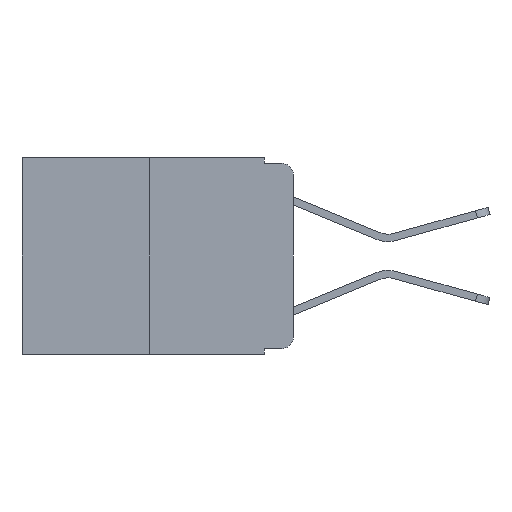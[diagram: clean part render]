
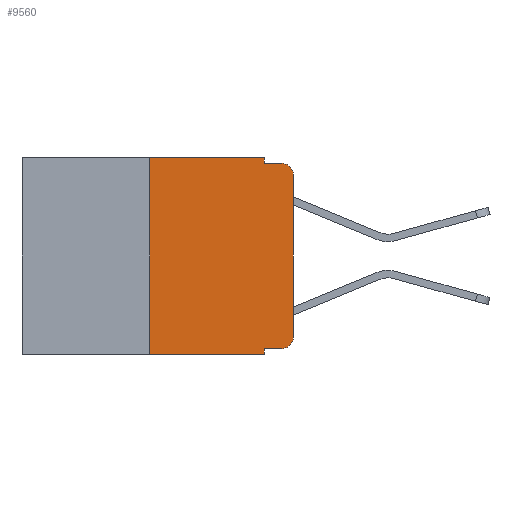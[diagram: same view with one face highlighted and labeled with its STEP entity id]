
A CAD part, left-side view. The second image highlights one B-rep face of the part: STEP entity #9560.
In plain terms, the highlighted planar face has unit normal (-1, 0, 0).
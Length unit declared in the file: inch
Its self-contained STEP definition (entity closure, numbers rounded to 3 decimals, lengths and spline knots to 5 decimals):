
#99 = VECTOR ( 'NONE', #3078, 39.37008 ) ;
#804 = DIRECTION ( 'NONE',  ( 0., -1., 0. ) ) ;
#1243 = ORIENTED_EDGE ( 'NONE', *, *, #24060, .F. ) ;
#1308 = CARTESIAN_POINT ( 'NONE',  ( 0., 0.473, 0. ) ) ;
#1434 = CARTESIAN_POINT ( 'NONE',  ( 0., 0.051, 0. ) ) ;
#1743 = DIRECTION ( 'NONE',  ( 0., 0., -1. ) ) ;
#1775 = DIRECTION ( 'NONE',  ( 0., 0., -1. ) ) ;
#1901 = ORIENTED_EDGE ( 'NONE', *, *, #14329, .F. ) ;
#2066 = VERTEX_POINT ( 'NONE', #2120 ) ;
#2120 = CARTESIAN_POINT ( 'NONE',  ( 0., 0.25, 0. ) ) ;
#2760 = PLANE ( 'NONE',  #17111 ) ;
#3078 = DIRECTION ( 'NONE',  ( 0., 0., 1. ) ) ;
#3568 = DIRECTION ( 'NONE',  ( -1., 0., 0. ) ) ;
#3966 = EDGE_CURVE ( 'NONE', #24525, #5085, #13087, .T. ) ;
#4762 = AXIS2_PLACEMENT_3D ( 'NONE', #24949, #13634, #1775 ) ;
#5085 = VERTEX_POINT ( 'NONE', #5779 ) ;
#5116 = LINE ( 'NONE', #18651, #10377 ) ;
#5595 = VERTEX_POINT ( 'NONE', #20746 ) ;
#5746 = VERTEX_POINT ( 'NONE', #14471 ) ;
#5779 = CARTESIAN_POINT ( 'NONE',  ( 0., 0.051, -0.343 ) ) ;
#5950 = VERTEX_POINT ( 'NONE', #19488 ) ;
#6272 = FACE_OUTER_BOUND ( 'NONE', #22135, .T. ) ;
#6300 = LINE ( 'NONE', #11685, #11519 ) ;
#6375 = LINE ( 'NONE', #20889, #21184 ) ;
#6711 = CARTESIAN_POINT ( 'NONE',  ( 0., 0.02, -0.03 ) ) ;
#6870 = DIRECTION ( 'NONE',  ( 0., 0., -1. ) ) ;
#6965 = DIRECTION ( 'NONE',  ( 0., -1., 0. ) ) ;
#7003 = EDGE_CURVE ( 'NONE', #5746, #5595, #13143, .T. ) ;
#7626 = CARTESIAN_POINT ( 'NONE',  ( 0., 0.25, -0.343 ) ) ;
#7671 = VERTEX_POINT ( 'NONE', #25083 ) ;
#7729 = EDGE_CURVE ( 'NONE', #18114, #5085, #6375, .T. ) ;
#7801 = EDGE_CURVE ( 'NONE', #21538, #5746, #5116, .T. ) ;
#7906 = ORIENTED_EDGE ( 'NONE', *, *, #7801, .T. ) ;
#7924 = VECTOR ( 'NONE', #15656, 39.37008 ) ;
#8271 = VERTEX_POINT ( 'NONE', #12628 ) ;
#8515 = ORIENTED_EDGE ( 'NONE', *, *, #7003, .T. ) ;
#8779 = CARTESIAN_POINT ( 'NONE',  ( 0., 0.051, -0.333 ) ) ;
#9560 = ADVANCED_FACE ( 'NONE', ( #6272 ), #2760, .F. ) ;
#9796 = CARTESIAN_POINT ( 'NONE',  ( 0., 0.051, 0. ) ) ;
#10217 = LINE ( 'NONE', #16835, #99 ) ;
#10377 = VECTOR ( 'NONE', #22731, 39.37008 ) ;
#10652 = ORIENTED_EDGE ( 'NONE', *, *, #15314, .T. ) ;
#11247 = ORIENTED_EDGE ( 'NONE', *, *, #7729, .T. ) ;
#11519 = VECTOR ( 'NONE', #21248, 39.37008 ) ;
#11596 = LINE ( 'NONE', #1308, #16732 ) ;
#11674 = EDGE_CURVE ( 'NONE', #18114, #2066, #10217, .T. ) ;
#11685 = CARTESIAN_POINT ( 'NONE',  ( 0., 0.051, -0.333 ) ) ;
#12448 = ORIENTED_EDGE ( 'NONE', *, *, #17003, .F. ) ;
#12628 = CARTESIAN_POINT ( 'NONE',  ( 0., 0.051, 0. ) ) ;
#12994 = CARTESIAN_POINT ( 'NONE',  ( 0., 0., -0.313 ) ) ;
#13010 = DIRECTION ( 'NONE',  ( 0., 0., -1. ) ) ;
#13087 = LINE ( 'NONE', #1434, #7924 ) ;
#13143 = CIRCLE ( 'NONE', #15792, 0.02 ) ;
#13466 = CIRCLE ( 'NONE', #4762, 0.02 ) ;
#13634 = DIRECTION ( 'NONE',  ( -1., 0., 0. ) ) ;
#14129 = VECTOR ( 'NONE', #804, 39.37008 ) ;
#14329 = EDGE_CURVE ( 'NONE', #7671, #5595, #24170, .T. ) ;
#14471 = CARTESIAN_POINT ( 'NONE',  ( 0., 0., -0.03 ) ) ;
#15148 = DIRECTION ( 'NONE',  ( 0., -1., 0. ) ) ;
#15176 = ORIENTED_EDGE ( 'NONE', *, *, #20413, .T. ) ;
#15314 = EDGE_CURVE ( 'NONE', #5950, #21538, #13466, .T. ) ;
#15656 = DIRECTION ( 'NONE',  ( 0., 0., -1. ) ) ;
#15792 = AXIS2_PLACEMENT_3D ( 'NONE', #6711, #3568, #13010 ) ;
#15807 = VECTOR ( 'NONE', #1743, 39.37008 ) ;
#16379 = ORIENTED_EDGE ( 'NONE', *, *, #3966, .F. ) ;
#16395 = LINE ( 'NONE', #9796, #15807 ) ;
#16538 = CARTESIAN_POINT ( 'NONE',  ( 0., 0.473, 0. ) ) ;
#16732 = VECTOR ( 'NONE', #15148, 39.37008 ) ;
#16835 = CARTESIAN_POINT ( 'NONE',  ( 0., 0.25, 0. ) ) ;
#16989 = ORIENTED_EDGE ( 'NONE', *, *, #11674, .F. ) ;
#17003 = EDGE_CURVE ( 'NONE', #8271, #7671, #16395, .T. ) ;
#17111 = AXIS2_PLACEMENT_3D ( 'NONE', #16538, #18481, #6870 ) ;
#18114 = VERTEX_POINT ( 'NONE', #7626 ) ;
#18481 = DIRECTION ( 'NONE',  ( 1., 0., 0. ) ) ;
#18651 = CARTESIAN_POINT ( 'NONE',  ( 0., 0., 0. ) ) ;
#19488 = CARTESIAN_POINT ( 'NONE',  ( 0., 0.02, -0.333 ) ) ;
#20413 = EDGE_CURVE ( 'NONE', #24525, #5950, #6300, .T. ) ;
#20746 = CARTESIAN_POINT ( 'NONE',  ( 0., 0.02, -0.01 ) ) ;
#20889 = CARTESIAN_POINT ( 'NONE',  ( 0., 0.473, -0.343 ) ) ;
#21184 = VECTOR ( 'NONE', #6965, 39.37008 ) ;
#21248 = DIRECTION ( 'NONE',  ( 0., -1., 0. ) ) ;
#21538 = VERTEX_POINT ( 'NONE', #12994 ) ;
#22135 = EDGE_LOOP ( 'NONE', ( #7906, #8515, #1901, #12448, #1243, #16989, #11247, #16379, #15176, #10652 ) ) ;
#22731 = DIRECTION ( 'NONE',  ( 0., 0., 1. ) ) ;
#24060 = EDGE_CURVE ( 'NONE', #2066, #8271, #11596, .T. ) ;
#24096 = CARTESIAN_POINT ( 'NONE',  ( 0., 0.051, -0.01 ) ) ;
#24170 = LINE ( 'NONE', #24096, #14129 ) ;
#24525 = VERTEX_POINT ( 'NONE', #8779 ) ;
#24949 = CARTESIAN_POINT ( 'NONE',  ( 0., 0.02, -0.313 ) ) ;
#25083 = CARTESIAN_POINT ( 'NONE',  ( 0., 0.051, -0.01 ) ) ;
